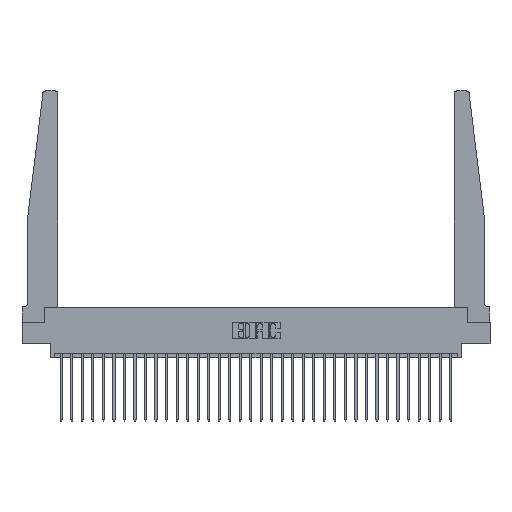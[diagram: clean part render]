
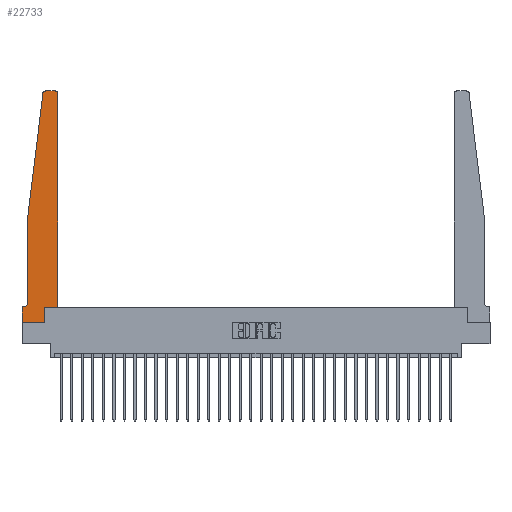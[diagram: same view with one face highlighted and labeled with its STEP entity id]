
A CAD part, top view. The second image highlights one B-rep face of the part: STEP entity #22733.
In plain terms, the highlighted planar face has unit normal (0, 0, 1).
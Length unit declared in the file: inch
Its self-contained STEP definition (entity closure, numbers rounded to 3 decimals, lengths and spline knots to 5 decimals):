
#416 = LINE ( 'NONE', #27229, #24559 ) ;
#434 = CARTESIAN_POINT ( 'NONE',  ( 0.395, 2.72, 0.37 ) ) ;
#502 = AXIS2_PLACEMENT_3D ( 'NONE', #434, #16826, #2767 ) ;
#1026 = CARTESIAN_POINT ( 'NONE',  ( 0., 0., 0.37 ) ) ;
#1244 = CARTESIAN_POINT ( 'NONE',  ( 0.27653, 2.72, 0.37 ) ) ;
#1739 = DIRECTION ( 'NONE',  ( 1., 0., 0. ) ) ;
#1774 = VERTEX_POINT ( 'NONE', #16174 ) ;
#2227 = CARTESIAN_POINT ( 'NONE',  ( 0.065, 0.2375, 0.37 ) ) ;
#2510 = VECTOR ( 'NONE', #14691, 39.37008 ) ;
#2511 = CARTESIAN_POINT ( 'NONE',  ( 0.065, 0.1875, 0.37 ) ) ;
#2767 = DIRECTION ( 'NONE',  ( 1., 0., 0. ) ) ;
#2834 = CARTESIAN_POINT ( 'NONE',  ( 0., 0.1875, 0.37 ) ) ;
#2853 = VECTOR ( 'NONE', #29216, 39.37008 ) ;
#2950 = CARTESIAN_POINT ( 'NONE',  ( 0.25, 2.75, 0.37 ) ) ;
#2975 = LINE ( 'NONE', #10020, #7777 ) ;
#3038 = CARTESIAN_POINT ( 'NONE',  ( 0.065, 1.25, 0.37 ) ) ;
#3411 = VECTOR ( 'NONE', #1739, 39.37008 ) ;
#3594 = DIRECTION ( 'NONE',  ( 1., 0., 0. ) ) ;
#3782 = VERTEX_POINT ( 'NONE', #18748 ) ;
#4094 = ORIENTED_EDGE ( 'NONE', *, *, #5862, .T. ) ;
#4345 = CARTESIAN_POINT ( 'NONE',  ( 0.27653, 2.75, 0.37 ) ) ;
#4393 = VERTEX_POINT ( 'NONE', #9066 ) ;
#4895 = DIRECTION ( 'NONE',  ( -1., 0., 0. ) ) ;
#5040 = VERTEX_POINT ( 'NONE', #14753 ) ;
#5160 = CIRCLE ( 'NONE', #22297, 0.05 ) ;
#5547 = ORIENTED_EDGE ( 'NONE', *, *, #13140, .T. ) ;
#5862 = EDGE_CURVE ( 'NONE', #17418, #11343, #17204, .T. ) ;
#6978 = CARTESIAN_POINT ( 'NONE',  ( 0.015, 0.2375, 0.37 ) ) ;
#7095 = ORIENTED_EDGE ( 'NONE', *, *, #25084, .T. ) ;
#7586 = LINE ( 'NONE', #18261, #12349 ) ;
#7777 = VECTOR ( 'NONE', #28696, 39.37008 ) ;
#7981 = EDGE_CURVE ( 'NONE', #21208, #19939, #17442, .T. ) ;
#9066 = CARTESIAN_POINT ( 'NONE',  ( 0.425, 2.72, 0.37 ) ) ;
#9095 = LINE ( 'NONE', #26863, #2853 ) ;
#9131 = EDGE_CURVE ( 'NONE', #24496, #5040, #7586, .T. ) ;
#9330 = DIRECTION ( 'NONE',  ( -1., 0., 0. ) ) ;
#10020 = CARTESIAN_POINT ( 'NONE',  ( 0.425, 0.18, 0.37 ) ) ;
#10734 = VECTOR ( 'NONE', #17791, 39.37008 ) ;
#10942 = EDGE_CURVE ( 'NONE', #11344, #24496, #26809, .T. ) ;
#10955 = PLANE ( 'NONE',  #22207 ) ;
#11204 = VECTOR ( 'NONE', #4895, 39.37008 ) ;
#11343 = VERTEX_POINT ( 'NONE', #26661 ) ;
#11344 = VERTEX_POINT ( 'NONE', #1026 ) ;
#11362 = CARTESIAN_POINT ( 'NONE',  ( 0.2605, 0., 0.37 ) ) ;
#11659 = LINE ( 'NONE', #27615, #16420 ) ;
#11687 = CIRCLE ( 'NONE', #502, 0.03 ) ;
#11948 = ORIENTED_EDGE ( 'NONE', *, *, #7981, .T. ) ;
#12211 = LINE ( 'NONE', #29399, #10734 ) ;
#12349 = VECTOR ( 'NONE', #13662, 39.37008 ) ;
#13140 = EDGE_CURVE ( 'NONE', #3782, #17418, #21232, .T. ) ;
#13662 = DIRECTION ( 'NONE',  ( 0., 1., 0. ) ) ;
#14249 = ORIENTED_EDGE ( 'NONE', *, *, #22110, .T. ) ;
#14346 = ORIENTED_EDGE ( 'NONE', *, *, #10942, .T. ) ;
#14592 = EDGE_CURVE ( 'NONE', #1774, #4393, #9095, .T. ) ;
#14691 = DIRECTION ( 'NONE',  ( -1., 0., 0. ) ) ;
#14753 = CARTESIAN_POINT ( 'NONE',  ( 0.2605, 0.18, 0.37 ) ) ;
#15672 = DIRECTION ( 'NONE',  ( 1., 0., 0. ) ) ;
#15798 = CARTESIAN_POINT ( 'NONE',  ( 0., 0., 0.37 ) ) ;
#16174 = CARTESIAN_POINT ( 'NONE',  ( 0.425, 0.18, 0.37 ) ) ;
#16237 = EDGE_CURVE ( 'NONE', #25506, #21208, #5160, .T. ) ;
#16420 = VECTOR ( 'NONE', #29973, 39.37008 ) ;
#16826 = DIRECTION ( 'NONE',  ( 0., 0., 1. ) ) ;
#17204 = CIRCLE ( 'NONE', #22923, 0.03 ) ;
#17418 = VERTEX_POINT ( 'NONE', #4345 ) ;
#17442 = LINE ( 'NONE', #2511, #11204 ) ;
#17644 = DIRECTION ( 'NONE',  ( 0., 0., 1. ) ) ;
#17791 = DIRECTION ( 'NONE',  ( -0.122, -0.992, 0. ) ) ;
#18104 = FACE_OUTER_BOUND ( 'NONE', #26413, .T. ) ;
#18228 = ORIENTED_EDGE ( 'NONE', *, *, #14592, .T. ) ;
#18261 = CARTESIAN_POINT ( 'NONE',  ( 0.2605, 0.18, 0.37 ) ) ;
#18748 = CARTESIAN_POINT ( 'NONE',  ( 0.395, 2.75, 0.37 ) ) ;
#19676 = ORIENTED_EDGE ( 'NONE', *, *, #16237, .T. ) ;
#19939 = VERTEX_POINT ( 'NONE', #2834 ) ;
#19976 = VERTEX_POINT ( 'NONE', #3038 ) ;
#20265 = CARTESIAN_POINT ( 'NONE',  ( 0., 0.1875, 0.37 ) ) ;
#20339 = DIRECTION ( 'NONE',  ( 0., -1., 0. ) ) ;
#21208 = VERTEX_POINT ( 'NONE', #23749 ) ;
#21232 = LINE ( 'NONE', #2950, #2510 ) ;
#22110 = EDGE_CURVE ( 'NONE', #11343, #19976, #12211, .T. ) ;
#22207 = AXIS2_PLACEMENT_3D ( 'NONE', #20265, #29627, #15672 ) ;
#22292 = ORIENTED_EDGE ( 'NONE', *, *, #30160, .T. ) ;
#22293 = ORIENTED_EDGE ( 'NONE', *, *, #24794, .T. ) ;
#22297 = AXIS2_PLACEMENT_3D ( 'NONE', #6978, #23339, #9330 ) ;
#22733 = ADVANCED_FACE ( 'NONE', ( #18104 ), #10955, .T. ) ;
#22923 = AXIS2_PLACEMENT_3D ( 'NONE', #1244, #17644, #3594 ) ;
#23339 = DIRECTION ( 'NONE',  ( 0., 0., -1. ) ) ;
#23749 = CARTESIAN_POINT ( 'NONE',  ( 0.015, 0.1875, 0.37 ) ) ;
#24496 = VERTEX_POINT ( 'NONE', #11362 ) ;
#24559 = VECTOR ( 'NONE', #20339, 39.37008 ) ;
#24794 = EDGE_CURVE ( 'NONE', #5040, #1774, #2975, .T. ) ;
#25084 = EDGE_CURVE ( 'NONE', #19976, #25506, #416, .T. ) ;
#25506 = VERTEX_POINT ( 'NONE', #2227 ) ;
#26413 = EDGE_LOOP ( 'NONE', ( #5547, #4094, #14249, #7095, #19676, #11948, #22292, #14346, #29178, #22293, #18228, #28262 ) ) ;
#26661 = CARTESIAN_POINT ( 'NONE',  ( 0.24675, 2.72367, 0.37 ) ) ;
#26794 = EDGE_CURVE ( 'NONE', #4393, #3782, #11687, .T. ) ;
#26809 = LINE ( 'NONE', #15798, #3411 ) ;
#26863 = CARTESIAN_POINT ( 'NONE',  ( 0.425, 0.18, 0.37 ) ) ;
#27229 = CARTESIAN_POINT ( 'NONE',  ( 0.065, 1.25, 0.37 ) ) ;
#27615 = CARTESIAN_POINT ( 'NONE',  ( 0., 0., 0.37 ) ) ;
#28262 = ORIENTED_EDGE ( 'NONE', *, *, #26794, .T. ) ;
#28696 = DIRECTION ( 'NONE',  ( 1., 0., 0. ) ) ;
#29178 = ORIENTED_EDGE ( 'NONE', *, *, #9131, .T. ) ;
#29216 = DIRECTION ( 'NONE',  ( 0., 1., 0. ) ) ;
#29399 = CARTESIAN_POINT ( 'NONE',  ( 0.065, 1.25, 0.37 ) ) ;
#29627 = DIRECTION ( 'NONE',  ( 0., 0., 1. ) ) ;
#29973 = DIRECTION ( 'NONE',  ( 0., -1., 0. ) ) ;
#30160 = EDGE_CURVE ( 'NONE', #19939, #11344, #11659, .T. ) ;
